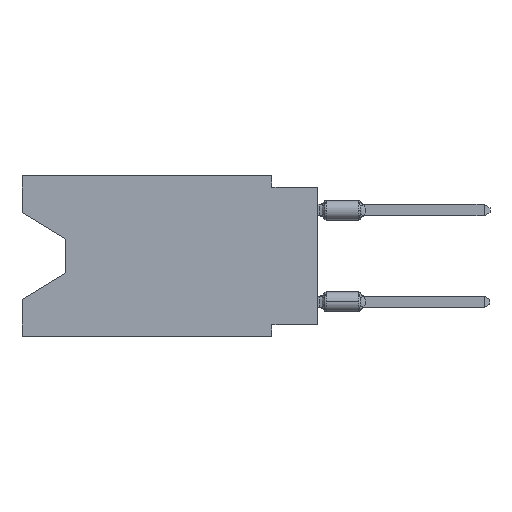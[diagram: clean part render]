
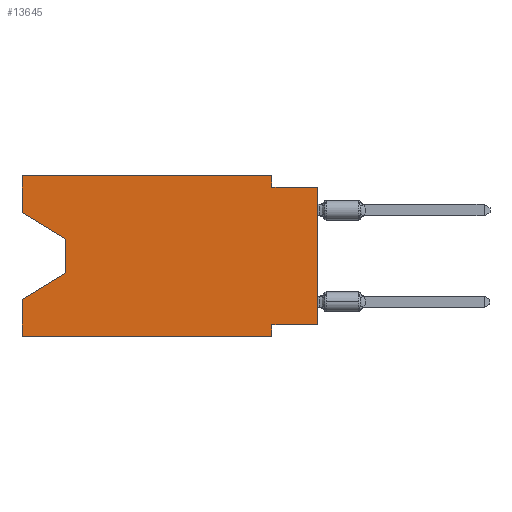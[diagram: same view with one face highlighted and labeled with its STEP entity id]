
A CAD part, left-side view. The second image highlights one B-rep face of the part: STEP entity #13645.
In plain terms, the highlighted planar face has unit normal (-1, 0, 0).
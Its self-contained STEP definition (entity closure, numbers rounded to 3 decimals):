
#65 = VERTEX_POINT ( 'NONE', #4490 ) ;
#285 = DIRECTION ( 'NONE',  ( 0., -1., 0. ) ) ;
#399 = ORIENTED_EDGE ( 'NONE', *, *, #11880, .T. ) ;
#758 = DIRECTION ( 'NONE',  ( 0., 0.855, -0.519 ) ) ;
#807 = CARTESIAN_POINT ( 'NONE',  ( 0., 16.383, -2.038 ) ) ;
#874 = DIRECTION ( 'NONE',  ( 1., 0., 0. ) ) ;
#910 = CARTESIAN_POINT ( 'NONE',  ( 0., 2.54, 0. ) ) ;
#938 = EDGE_CURVE ( 'NONE', #10750, #1023, #5751, .T. ) ;
#969 = LINE ( 'NONE', #10572, #10224 ) ;
#1002 = VERTEX_POINT ( 'NONE', #10438 ) ;
#1023 = VERTEX_POINT ( 'NONE', #4089 ) ;
#1212 = VERTEX_POINT ( 'NONE', #7537 ) ;
#1238 = EDGE_CURVE ( 'NONE', #65, #1002, #13194, .T. ) ;
#1254 = EDGE_CURVE ( 'NONE', #10750, #7891, #2630, .T. ) ;
#2145 = EDGE_CURVE ( 'NONE', #12584, #9571, #6851, .T. ) ;
#2151 = LINE ( 'NONE', #910, #12382 ) ;
#2363 = EDGE_CURVE ( 'NONE', #10723, #8558, #2151, .T. ) ;
#2572 = EDGE_CURVE ( 'NONE', #6995, #1002, #12142, .T. ) ;
#2630 = LINE ( 'NONE', #3589, #3851 ) ;
#2644 = CARTESIAN_POINT ( 'NONE',  ( 0., 0., 0. ) ) ;
#2678 = CARTESIAN_POINT ( 'NONE',  ( 0., 16.383, 0. ) ) ;
#2808 = VECTOR ( 'NONE', #10096, 1000. ) ;
#3205 = DIRECTION ( 'NONE',  ( 0., 0., -1. ) ) ;
#3316 = CARTESIAN_POINT ( 'NONE',  ( 0., 16.383, 0. ) ) ;
#3451 = ORIENTED_EDGE ( 'NONE', *, *, #2145, .F. ) ;
#3537 = ORIENTED_EDGE ( 'NONE', *, *, #1254, .F. ) ;
#3589 = CARTESIAN_POINT ( 'NONE',  ( 0., 0., -8.255 ) ) ;
#3851 = VECTOR ( 'NONE', #6782, 1000. ) ;
#3961 = DIRECTION ( 'NONE',  ( 0., -1., 0. ) ) ;
#3968 = CARTESIAN_POINT ( 'NONE',  ( 0., 2.54, -8.255 ) ) ;
#3973 = DIRECTION ( 'NONE',  ( 0., 0., -1. ) ) ;
#4089 = CARTESIAN_POINT ( 'NONE',  ( 0., 0., -0.635 ) ) ;
#4280 = CARTESIAN_POINT ( 'NONE',  ( 0., 2.54, 0. ) ) ;
#4469 = ORIENTED_EDGE ( 'NONE', *, *, #2572, .T. ) ;
#4490 = CARTESIAN_POINT ( 'NONE',  ( 0., 16.383, -8.89 ) ) ;
#4769 = DIRECTION ( 'NONE',  ( 0., 0., 1. ) ) ;
#4931 = ORIENTED_EDGE ( 'NONE', *, *, #13038, .T. ) ;
#4973 = VECTOR ( 'NONE', #285, 1000. ) ;
#5181 = DIRECTION ( 'NONE',  ( 0., -1., 0. ) ) ;
#5301 = ORIENTED_EDGE ( 'NONE', *, *, #13120, .F. ) ;
#5396 = VECTOR ( 'NONE', #13225, 1000. ) ;
#5664 = EDGE_LOOP ( 'NONE', ( #399, #10067, #4469, #12514, #4931, #5301, #3537, #12817, #12046, #9520, #12302, #3451 ) ) ;
#5751 = LINE ( 'NONE', #2644, #12297 ) ;
#5868 = VECTOR ( 'NONE', #3961, 1000. ) ;
#5885 = CARTESIAN_POINT ( 'NONE',  ( 0., 16.383, 0. ) ) ;
#5965 = CARTESIAN_POINT ( 'NONE',  ( 0., 16.383, -8.89 ) ) ;
#5973 = CARTESIAN_POINT ( 'NONE',  ( 0., 13.97, -3.505 ) ) ;
#6291 = VECTOR ( 'NONE', #758, 1000. ) ;
#6308 = LINE ( 'NONE', #6377, #7846 ) ;
#6377 = CARTESIAN_POINT ( 'NONE',  ( 0., 2.54, -8.89 ) ) ;
#6730 = CARTESIAN_POINT ( 'NONE',  ( 0., 13.97, -3.505 ) ) ;
#6782 = DIRECTION ( 'NONE',  ( 0., 1., 0. ) ) ;
#6851 = LINE ( 'NONE', #5885, #2808 ) ;
#6995 = VERTEX_POINT ( 'NONE', #9261 ) ;
#7210 = CARTESIAN_POINT ( 'NONE',  ( 0., 16.383, -2.038 ) ) ;
#7537 = CARTESIAN_POINT ( 'NONE',  ( 0., 2.54, -8.89 ) ) ;
#7826 = EDGE_CURVE ( 'NONE', #12804, #6995, #9021, .T. ) ;
#7846 = VECTOR ( 'NONE', #3205, 1000. ) ;
#7891 = VERTEX_POINT ( 'NONE', #3968 ) ;
#8308 = VECTOR ( 'NONE', #9545, 1000. ) ;
#8518 = LINE ( 'NONE', #8792, #4973 ) ;
#8558 = VERTEX_POINT ( 'NONE', #11105 ) ;
#8792 = CARTESIAN_POINT ( 'NONE',  ( 0., 16.383, 0. ) ) ;
#8849 = CARTESIAN_POINT ( 'NONE',  ( 0., 16.383, 0. ) ) ;
#9021 = LINE ( 'NONE', #5973, #5396 ) ;
#9216 = LINE ( 'NONE', #5965, #5868 ) ;
#9261 = CARTESIAN_POINT ( 'NONE',  ( 0., 13.97, -5.385 ) ) ;
#9292 = FACE_OUTER_BOUND ( 'NONE', #5664, .T. ) ;
#9520 = ORIENTED_EDGE ( 'NONE', *, *, #2363, .F. ) ;
#9545 = DIRECTION ( 'NONE',  ( 0., -0.855, -0.519 ) ) ;
#9571 = VERTEX_POINT ( 'NONE', #3316 ) ;
#10036 = DIRECTION ( 'NONE',  ( 0., 0., 1. ) ) ;
#10067 = ORIENTED_EDGE ( 'NONE', *, *, #7826, .T. ) ;
#10096 = DIRECTION ( 'NONE',  ( 0., 0., 1. ) ) ;
#10224 = VECTOR ( 'NONE', #5181, 1000. ) ;
#10438 = CARTESIAN_POINT ( 'NONE',  ( 0., 16.383, -6.852 ) ) ;
#10572 = CARTESIAN_POINT ( 'NONE',  ( 0., 0., -0.635 ) ) ;
#10697 = EDGE_CURVE ( 'NONE', #8558, #1023, #969, .T. ) ;
#10723 = VERTEX_POINT ( 'NONE', #4280 ) ;
#10750 = VERTEX_POINT ( 'NONE', #13610 ) ;
#11043 = CARTESIAN_POINT ( 'NONE',  ( 0., 13.97, -5.385 ) ) ;
#11105 = CARTESIAN_POINT ( 'NONE',  ( 0., 2.54, -0.635 ) ) ;
#11341 = LINE ( 'NONE', #7210, #8308 ) ;
#11471 = DIRECTION ( 'NONE',  ( 0., 0., -1. ) ) ;
#11880 = EDGE_CURVE ( 'NONE', #12584, #12804, #11341, .T. ) ;
#12031 = EDGE_CURVE ( 'NONE', #9571, #10723, #8518, .T. ) ;
#12046 = ORIENTED_EDGE ( 'NONE', *, *, #10697, .F. ) ;
#12142 = LINE ( 'NONE', #11043, #6291 ) ;
#12297 = VECTOR ( 'NONE', #10036, 1000. ) ;
#12302 = ORIENTED_EDGE ( 'NONE', *, *, #12031, .F. ) ;
#12382 = VECTOR ( 'NONE', #11471, 1000. ) ;
#12465 = PLANE ( 'NONE',  #13148 ) ;
#12514 = ORIENTED_EDGE ( 'NONE', *, *, #1238, .F. ) ;
#12584 = VERTEX_POINT ( 'NONE', #807 ) ;
#12670 = VECTOR ( 'NONE', #4769, 1000. ) ;
#12804 = VERTEX_POINT ( 'NONE', #6730 ) ;
#12817 = ORIENTED_EDGE ( 'NONE', *, *, #938, .T. ) ;
#13038 = EDGE_CURVE ( 'NONE', #65, #1212, #9216, .T. ) ;
#13120 = EDGE_CURVE ( 'NONE', #7891, #1212, #6308, .T. ) ;
#13148 = AXIS2_PLACEMENT_3D ( 'NONE', #2678, #874, #3973 ) ;
#13194 = LINE ( 'NONE', #8849, #12670 ) ;
#13225 = DIRECTION ( 'NONE',  ( 0., 0., -1. ) ) ;
#13610 = CARTESIAN_POINT ( 'NONE',  ( 0., 0., -8.255 ) ) ;
#13645 = ADVANCED_FACE ( 'NONE', ( #9292 ), #12465, .F. ) ;
